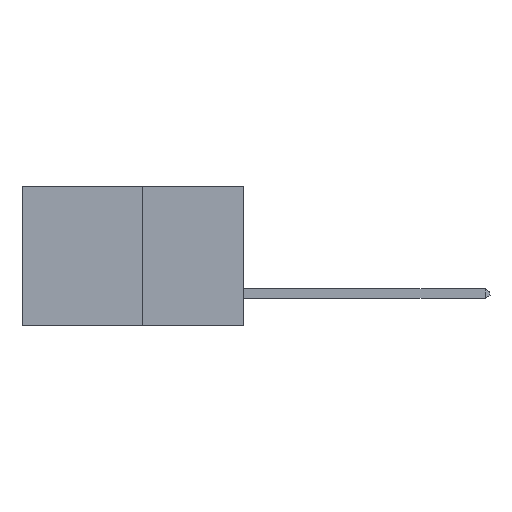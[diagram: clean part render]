
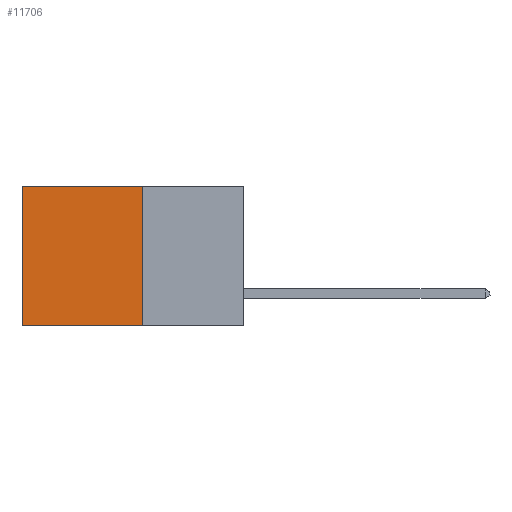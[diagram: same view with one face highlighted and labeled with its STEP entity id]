
A CAD part, left-side view. The second image highlights one B-rep face of the part: STEP entity #11706.
In plain terms, the highlighted planar face has unit normal (-1, 0, 0).
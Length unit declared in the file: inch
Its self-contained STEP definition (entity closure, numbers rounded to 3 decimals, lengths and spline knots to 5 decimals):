
#648 = LINE ( 'NONE', #4390, #2940 ) ;
#687 = VERTEX_POINT ( 'NONE', #11969 ) ;
#890 = DIRECTION ( 'NONE',  ( 0., 1., 0. ) ) ;
#918 = EDGE_LOOP ( 'NONE', ( #4160, #11925, #6746, #9765 ) ) ;
#1575 = CARTESIAN_POINT ( 'NONE',  ( 0.277, 0.27, -0.37 ) ) ;
#1980 = VECTOR ( 'NONE', #11317, 39.37008 ) ;
#2474 = EDGE_CURVE ( 'NONE', #687, #9624, #648, .T. ) ;
#2940 = VECTOR ( 'NONE', #890, 39.37008 ) ;
#3516 = EDGE_CURVE ( 'NONE', #687, #9309, #8328, .T. ) ;
#3605 = DIRECTION ( 'NONE',  ( 0., 0., -1. ) ) ;
#3808 = CARTESIAN_POINT ( 'NONE',  ( 0.277, 0.27, -0.37 ) ) ;
#3940 = VECTOR ( 'NONE', #8198, 39.37008 ) ;
#3999 = DIRECTION ( 'NONE',  ( 1., 0., 0. ) ) ;
#4093 = LINE ( 'NONE', #9214, #6547 ) ;
#4160 = ORIENTED_EDGE ( 'NONE', *, *, #11414, .T. ) ;
#4390 = CARTESIAN_POINT ( 'NONE',  ( 0.277, 0.27, 0. ) ) ;
#5274 = CARTESIAN_POINT ( 'NONE',  ( 0.277, 0.27, -0.37 ) ) ;
#6547 = VECTOR ( 'NONE', #3605, 39.37008 ) ;
#6746 = ORIENTED_EDGE ( 'NONE', *, *, #3516, .F. ) ;
#6938 = CARTESIAN_POINT ( 'NONE',  ( 0.277, 0.59, 0. ) ) ;
#7589 = LINE ( 'NONE', #3808, #1980 ) ;
#8031 = FACE_OUTER_BOUND ( 'NONE', #918, .T. ) ;
#8198 = DIRECTION ( 'NONE',  ( 0., 0., -1. ) ) ;
#8328 = LINE ( 'NONE', #1575, #3940 ) ;
#8779 = AXIS2_PLACEMENT_3D ( 'NONE', #9590, #3999, #10585 ) ;
#9214 = CARTESIAN_POINT ( 'NONE',  ( 0.277, 0.59, -0.37 ) ) ;
#9309 = VERTEX_POINT ( 'NONE', #5274 ) ;
#9555 = VERTEX_POINT ( 'NONE', #11509 ) ;
#9590 = CARTESIAN_POINT ( 'NONE',  ( 0.277, 0.27, -0.37 ) ) ;
#9624 = VERTEX_POINT ( 'NONE', #6938 ) ;
#9765 = ORIENTED_EDGE ( 'NONE', *, *, #2474, .T. ) ;
#10585 = DIRECTION ( 'NONE',  ( 0., 0., -1. ) ) ;
#11317 = DIRECTION ( 'NONE',  ( 0., 1., 0. ) ) ;
#11414 = EDGE_CURVE ( 'NONE', #9624, #9555, #4093, .T. ) ;
#11437 = PLANE ( 'NONE',  #8779 ) ;
#11509 = CARTESIAN_POINT ( 'NONE',  ( 0.277, 0.59, -0.37 ) ) ;
#11586 = EDGE_CURVE ( 'NONE', #9309, #9555, #7589, .T. ) ;
#11706 = ADVANCED_FACE ( 'NONE', ( #8031 ), #11437, .F. ) ;
#11925 = ORIENTED_EDGE ( 'NONE', *, *, #11586, .F. ) ;
#11969 = CARTESIAN_POINT ( 'NONE',  ( 0.277, 0.27, 0. ) ) ;
